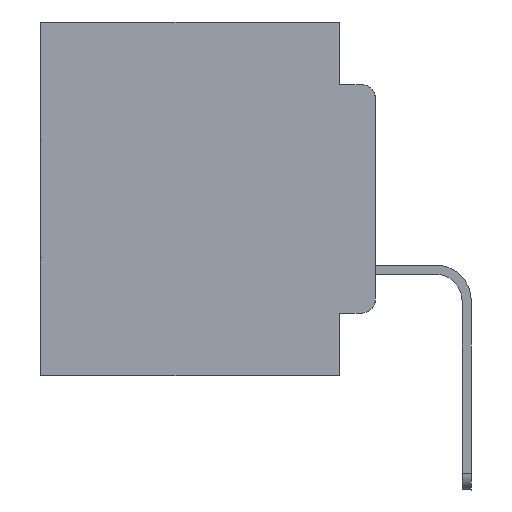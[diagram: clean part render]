
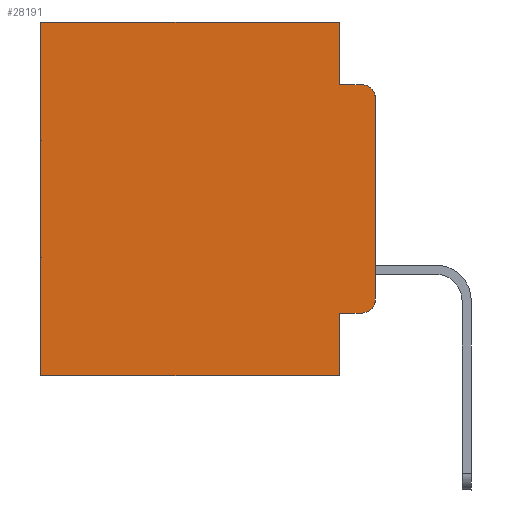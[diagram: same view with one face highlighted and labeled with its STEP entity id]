
A CAD part, left-side view. The second image highlights one B-rep face of the part: STEP entity #28191.
In plain terms, the highlighted planar face has unit normal (-1, 0, 0).
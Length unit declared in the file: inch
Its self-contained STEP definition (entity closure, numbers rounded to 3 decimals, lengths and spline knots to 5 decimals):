
#20 = CIRCLE ( 'NONE', #3769, 0.02 ) ;
#92 = CARTESIAN_POINT ( 'NONE',  ( 0.298, 0.02, -0.0885 ) ) ;
#833 = LINE ( 'NONE', #25808, #12764 ) ;
#1048 = CARTESIAN_POINT ( 'NONE',  ( 0.298, 0.051, 0. ) ) ;
#1312 = DIRECTION ( 'NONE',  ( 0., -1., 0. ) ) ;
#1702 = CARTESIAN_POINT ( 'NONE',  ( 0.298, 0.051, -0.0885 ) ) ;
#2400 = CARTESIAN_POINT ( 'NONE',  ( 0.298, 0., 0. ) ) ;
#2476 = CARTESIAN_POINT ( 'NONE',  ( 0.298, 0.473, 0. ) ) ;
#3071 = LINE ( 'NONE', #12359, #20066 ) ;
#3769 = AXIS2_PLACEMENT_3D ( 'NONE', #26308, #19649, #10160 ) ;
#4533 = CARTESIAN_POINT ( 'NONE',  ( 0.298, 0., 0. ) ) ;
#4712 = DIRECTION ( 'NONE',  ( 1., 0., 0. ) ) ;
#4878 = DIRECTION ( 'NONE',  ( 0., 1., 0. ) ) ;
#5097 = AXIS2_PLACEMENT_3D ( 'NONE', #10119, #14779, #26253 ) ;
#5129 = VERTEX_POINT ( 'NONE', #10297 ) ;
#5754 = VERTEX_POINT ( 'NONE', #23106 ) ;
#6028 = AXIS2_PLACEMENT_3D ( 'NONE', #2400, #4712, #23246 ) ;
#6107 = CARTESIAN_POINT ( 'NONE',  ( 0.298, 0.473, -0.5 ) ) ;
#6359 = EDGE_CURVE ( 'NONE', #8116, #12724, #14785, .T. ) ;
#6423 = CARTESIAN_POINT ( 'NONE',  ( 0.298, 0.051, -0.5 ) ) ;
#7308 = CARTESIAN_POINT ( 'NONE',  ( 0.298, 0., -0.3915 ) ) ;
#7928 = CARTESIAN_POINT ( 'NONE',  ( 0.298, 0.051, 0. ) ) ;
#8116 = VERTEX_POINT ( 'NONE', #25928 ) ;
#9333 = VERTEX_POINT ( 'NONE', #6423 ) ;
#9666 = VERTEX_POINT ( 'NONE', #2476 ) ;
#9686 = EDGE_CURVE ( 'NONE', #25593, #9666, #833, .T. ) ;
#10010 = ORIENTED_EDGE ( 'NONE', *, *, #14172, .T. ) ;
#10119 = CARTESIAN_POINT ( 'NONE',  ( 0.298, 0.02, -0.3915 ) ) ;
#10160 = DIRECTION ( 'NONE',  ( 0., 0., -1. ) ) ;
#10297 = CARTESIAN_POINT ( 'NONE',  ( 0.298, 0.051, -0.0885 ) ) ;
#10331 = DIRECTION ( 'NONE',  ( 0., 0., -1. ) ) ;
#10569 = VECTOR ( 'NONE', #12688, 39.37008 ) ;
#10663 = VECTOR ( 'NONE', #1312, 39.37008 ) ;
#12359 = CARTESIAN_POINT ( 'NONE',  ( 0.298, 0.051, -0.4115 ) ) ;
#12544 = ORIENTED_EDGE ( 'NONE', *, *, #19131, .F. ) ;
#12688 = DIRECTION ( 'NONE',  ( 0., 0., -1. ) ) ;
#12724 = VERTEX_POINT ( 'NONE', #7308 ) ;
#12764 = VECTOR ( 'NONE', #4878, 39.37008 ) ;
#12769 = EDGE_CURVE ( 'NONE', #5754, #12724, #23810, .T. ) ;
#12873 = LINE ( 'NONE', #17412, #19419 ) ;
#12920 = CARTESIAN_POINT ( 'NONE',  ( 0.298, 0., -0.5 ) ) ;
#13126 = ORIENTED_EDGE ( 'NONE', *, *, #14127, .F. ) ;
#13602 = ORIENTED_EDGE ( 'NONE', *, *, #9686, .T. ) ;
#13989 = ORIENTED_EDGE ( 'NONE', *, *, #6359, .F. ) ;
#14127 = EDGE_CURVE ( 'NONE', #25593, #5129, #15406, .T. ) ;
#14172 = EDGE_CURVE ( 'NONE', #20984, #5754, #3071, .T. ) ;
#14239 = CARTESIAN_POINT ( 'NONE',  ( 0.298, 0.051, 0. ) ) ;
#14779 = DIRECTION ( 'NONE',  ( -1., 0., 0. ) ) ;
#14785 = LINE ( 'NONE', #4533, #20192 ) ;
#15406 = LINE ( 'NONE', #7928, #27663 ) ;
#15602 = VERTEX_POINT ( 'NONE', #6107 ) ;
#16281 = PLANE ( 'NONE',  #6028 ) ;
#17412 = CARTESIAN_POINT ( 'NONE',  ( 0.298, 0.473, 0. ) ) ;
#19131 = EDGE_CURVE ( 'NONE', #5129, #23061, #29816, .T. ) ;
#19246 = DIRECTION ( 'NONE',  ( 0., -1., 0. ) ) ;
#19419 = VECTOR ( 'NONE', #10331, 39.37008 ) ;
#19649 = DIRECTION ( 'NONE',  ( -1., 0., 0. ) ) ;
#19836 = EDGE_LOOP ( 'NONE', ( #13989, #24121, #12544, #13126, #13602, #24351, #20930, #22351, #10010, #27486 ) ) ;
#20066 = VECTOR ( 'NONE', #19246, 39.37008 ) ;
#20192 = VECTOR ( 'NONE', #20712, 39.37008 ) ;
#20583 = EDGE_CURVE ( 'NONE', #8116, #23061, #20, .T. ) ;
#20712 = DIRECTION ( 'NONE',  ( 0., 0., -1. ) ) ;
#20803 = LINE ( 'NONE', #12920, #23012 ) ;
#20930 = ORIENTED_EDGE ( 'NONE', *, *, #27905, .F. ) ;
#20984 = VERTEX_POINT ( 'NONE', #21454 ) ;
#21454 = CARTESIAN_POINT ( 'NONE',  ( 0.298, 0.051, -0.4115 ) ) ;
#21496 = FACE_OUTER_BOUND ( 'NONE', #19836, .T. ) ;
#22351 = ORIENTED_EDGE ( 'NONE', *, *, #23908, .F. ) ;
#23012 = VECTOR ( 'NONE', #24566, 39.37008 ) ;
#23061 = VERTEX_POINT ( 'NONE', #92 ) ;
#23106 = CARTESIAN_POINT ( 'NONE',  ( 0.298, 0.02, -0.4115 ) ) ;
#23246 = DIRECTION ( 'NONE',  ( 0., 0., -1. ) ) ;
#23810 = CIRCLE ( 'NONE', #5097, 0.02 ) ;
#23908 = EDGE_CURVE ( 'NONE', #20984, #9333, #26794, .T. ) ;
#24121 = ORIENTED_EDGE ( 'NONE', *, *, #20583, .T. ) ;
#24351 = ORIENTED_EDGE ( 'NONE', *, *, #27286, .T. ) ;
#24566 = DIRECTION ( 'NONE',  ( 0., 1., 0. ) ) ;
#25593 = VERTEX_POINT ( 'NONE', #14239 ) ;
#25808 = CARTESIAN_POINT ( 'NONE',  ( 0.298, 0., 0. ) ) ;
#25928 = CARTESIAN_POINT ( 'NONE',  ( 0.298, 0., -0.1085 ) ) ;
#26253 = DIRECTION ( 'NONE',  ( 0., 0., -1. ) ) ;
#26308 = CARTESIAN_POINT ( 'NONE',  ( 0.298, 0.02, -0.1085 ) ) ;
#26794 = LINE ( 'NONE', #1048, #10569 ) ;
#27286 = EDGE_CURVE ( 'NONE', #9666, #15602, #12873, .T. ) ;
#27486 = ORIENTED_EDGE ( 'NONE', *, *, #12769, .T. ) ;
#27663 = VECTOR ( 'NONE', #28840, 39.37008 ) ;
#27905 = EDGE_CURVE ( 'NONE', #9333, #15602, #20803, .T. ) ;
#28191 = ADVANCED_FACE ( 'NONE', ( #21496 ), #16281, .F. ) ;
#28840 = DIRECTION ( 'NONE',  ( 0., 0., -1. ) ) ;
#29816 = LINE ( 'NONE', #1702, #10663 ) ;
